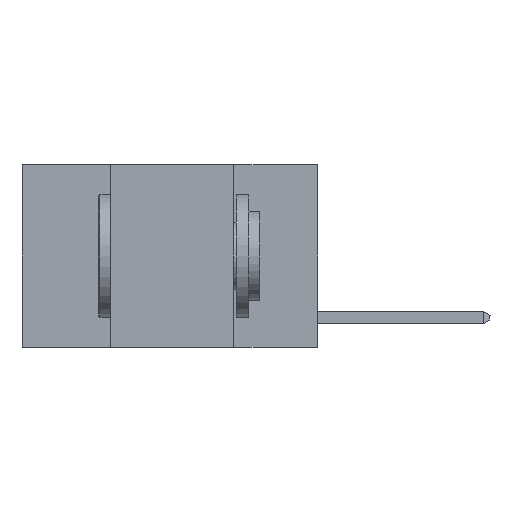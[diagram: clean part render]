
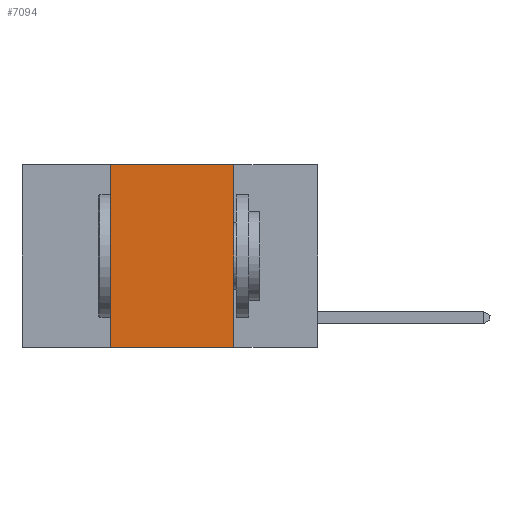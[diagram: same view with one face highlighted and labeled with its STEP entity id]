
A CAD part, left-side view. The second image highlights one B-rep face of the part: STEP entity #7094.
In plain terms, the highlighted planar face has unit normal (-1, 0, 0).
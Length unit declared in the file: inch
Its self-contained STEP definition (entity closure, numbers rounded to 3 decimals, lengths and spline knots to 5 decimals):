
#72 = VECTOR ( 'NONE', #8587, 39.37008 ) ;
#248 = VERTEX_POINT ( 'NONE', #7181 ) ;
#286 = CARTESIAN_POINT ( 'NONE',  ( 0., 0.42, 0. ) ) ;
#321 = EDGE_CURVE ( 'NONE', #248, #5312, #6064, .T. ) ;
#353 = LINE ( 'NONE', #286, #8997 ) ;
#360 = EDGE_LOOP ( 'NONE', ( #10239, #9602, #7906, #10441 ) ) ;
#565 = CARTESIAN_POINT ( 'NONE',  ( 0., 0.6, 0. ) ) ;
#1057 = DIRECTION ( 'NONE',  ( 0., 0., -1. ) ) ;
#1754 = AXIS2_PLACEMENT_3D ( 'NONE', #1914, #5456, #8941 ) ;
#1914 = CARTESIAN_POINT ( 'NONE',  ( 0., 0.6, 0. ) ) ;
#2523 = CARTESIAN_POINT ( 'NONE',  ( 0., 0.42, 0. ) ) ;
#3150 = VECTOR ( 'NONE', #5911, 39.37008 ) ;
#3154 = VERTEX_POINT ( 'NONE', #7462 ) ;
#4326 = VECTOR ( 'NONE', #1057, 39.37008 ) ;
#4671 = DIRECTION ( 'NONE',  ( 0., 0., 1. ) ) ;
#4696 = VERTEX_POINT ( 'NONE', #2523 ) ;
#4868 = EDGE_CURVE ( 'NONE', #3154, #4696, #353, .T. ) ;
#5312 = VERTEX_POINT ( 'NONE', #5637 ) ;
#5369 = EDGE_CURVE ( 'NONE', #4696, #248, #6703, .T. ) ;
#5456 = DIRECTION ( 'NONE',  ( 1., 0., 0. ) ) ;
#5475 = EDGE_CURVE ( 'NONE', #3154, #5312, #6579, .T. ) ;
#5637 = CARTESIAN_POINT ( 'NONE',  ( 0., 0.17, -0.37 ) ) ;
#5911 = DIRECTION ( 'NONE',  ( 0., -1., 0. ) ) ;
#6064 = LINE ( 'NONE', #7127, #4326 ) ;
#6241 = FACE_OUTER_BOUND ( 'NONE', #360, .T. ) ;
#6579 = LINE ( 'NONE', #10092, #72 ) ;
#6703 = LINE ( 'NONE', #565, #3150 ) ;
#7094 = ADVANCED_FACE ( 'NONE', ( #6241 ), #9749, .F. ) ;
#7127 = CARTESIAN_POINT ( 'NONE',  ( 0., 0.17, 0. ) ) ;
#7181 = CARTESIAN_POINT ( 'NONE',  ( 0., 0.17, 0. ) ) ;
#7462 = CARTESIAN_POINT ( 'NONE',  ( 0., 0.42, -0.37 ) ) ;
#7906 = ORIENTED_EDGE ( 'NONE', *, *, #4868, .F. ) ;
#8587 = DIRECTION ( 'NONE',  ( 0., -1., 0. ) ) ;
#8941 = DIRECTION ( 'NONE',  ( 0., 0., -1. ) ) ;
#8997 = VECTOR ( 'NONE', #4671, 39.37008 ) ;
#9602 = ORIENTED_EDGE ( 'NONE', *, *, #5369, .F. ) ;
#9749 = PLANE ( 'NONE',  #1754 ) ;
#10092 = CARTESIAN_POINT ( 'NONE',  ( 0., 0.6, -0.37 ) ) ;
#10239 = ORIENTED_EDGE ( 'NONE', *, *, #321, .F. ) ;
#10441 = ORIENTED_EDGE ( 'NONE', *, *, #5475, .T. ) ;
